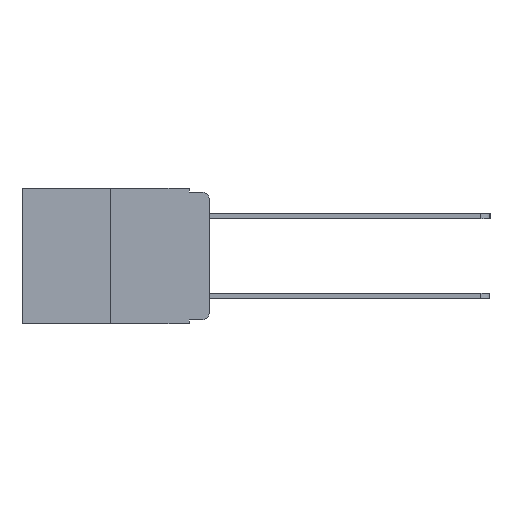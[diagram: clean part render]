
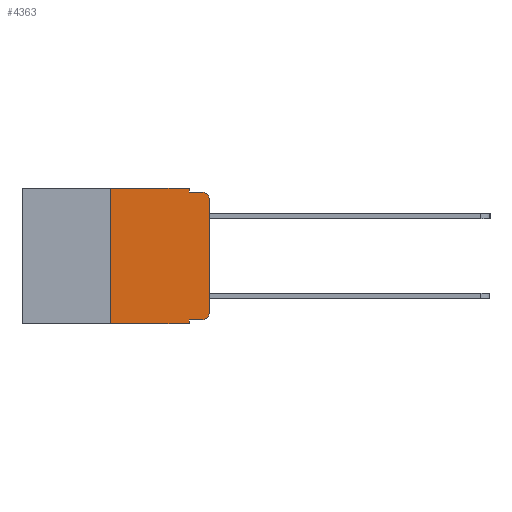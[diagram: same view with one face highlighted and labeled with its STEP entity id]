
A CAD part, left-side view. The second image highlights one B-rep face of the part: STEP entity #4363.
In plain terms, the highlighted planar face has unit normal (-1, 0, 0).
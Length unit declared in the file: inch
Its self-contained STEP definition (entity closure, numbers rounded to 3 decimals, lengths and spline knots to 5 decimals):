
#82 = VECTOR ( 'NONE', #4408, 39.37008 ) ;
#122 = EDGE_CURVE ( 'NONE', #7016, #6286, #2641, .T. ) ;
#457 = ORIENTED_EDGE ( 'NONE', *, *, #4358, .F. ) ;
#758 = ORIENTED_EDGE ( 'NONE', *, *, #6262, .T. ) ;
#801 = EDGE_CURVE ( 'NONE', #7571, #7016, #3825, .T. ) ;
#914 = PLANE ( 'NONE',  #8276 ) ;
#931 = LINE ( 'NONE', #12669, #4138 ) ;
#958 = VECTOR ( 'NONE', #11687, 39.37008 ) ;
#1059 = CARTESIAN_POINT ( 'NONE',  ( 0., 0.02, -0.01 ) ) ;
#1319 = CARTESIAN_POINT ( 'NONE',  ( 0., 0.051, -0.01 ) ) ;
#1342 = CARTESIAN_POINT ( 'NONE',  ( 0., 0.051, 0. ) ) ;
#1504 = EDGE_CURVE ( 'NONE', #7571, #2391, #10440, .T. ) ;
#1581 = CARTESIAN_POINT ( 'NONE',  ( 0., 0.051, -0.333 ) ) ;
#1726 = CARTESIAN_POINT ( 'NONE',  ( 0., 0.02, -0.333 ) ) ;
#2180 = CARTESIAN_POINT ( 'NONE',  ( 0., 0.051, -0.333 ) ) ;
#2243 = EDGE_CURVE ( 'NONE', #11207, #2372, #931, .T. ) ;
#2277 = ORIENTED_EDGE ( 'NONE', *, *, #5172, .T. ) ;
#2372 = VERTEX_POINT ( 'NONE', #4711 ) ;
#2391 = VERTEX_POINT ( 'NONE', #11689 ) ;
#2641 = CIRCLE ( 'NONE', #10747, 0.02 ) ;
#2781 = VECTOR ( 'NONE', #5184, 39.37008 ) ;
#2895 = LINE ( 'NONE', #3265, #82 ) ;
#2938 = ORIENTED_EDGE ( 'NONE', *, *, #2961, .F. ) ;
#2961 = EDGE_CURVE ( 'NONE', #12377, #11466, #12189, .T. ) ;
#3074 = DIRECTION ( 'NONE',  ( 1., 0., 0. ) ) ;
#3123 = DIRECTION ( 'NONE',  ( 0., 0., -1. ) ) ;
#3153 = DIRECTION ( 'NONE',  ( -1., 0., 0. ) ) ;
#3265 = CARTESIAN_POINT ( 'NONE',  ( 0., 0., 0. ) ) ;
#3700 = EDGE_CURVE ( 'NONE', #11466, #9908, #11582, .T. ) ;
#3782 = VECTOR ( 'NONE', #8153, 39.37008 ) ;
#3808 = CARTESIAN_POINT ( 'NONE',  ( 0., 0., -0.313 ) ) ;
#3825 = LINE ( 'NONE', #2180, #958 ) ;
#3977 = AXIS2_PLACEMENT_3D ( 'NONE', #5525, #12126, #6501 ) ;
#4138 = VECTOR ( 'NONE', #12748, 39.37008 ) ;
#4358 = EDGE_CURVE ( 'NONE', #2372, #12377, #11291, .T. ) ;
#4363 = ADVANCED_FACE ( 'NONE', ( #6256 ), #914, .F. ) ;
#4408 = DIRECTION ( 'NONE',  ( 0., 0., 1. ) ) ;
#4439 = EDGE_CURVE ( 'NONE', #6180, #9908, #9840, .T. ) ;
#4711 = CARTESIAN_POINT ( 'NONE',  ( 0., 0.25, 0. ) ) ;
#5172 = EDGE_CURVE ( 'NONE', #6286, #6180, #2895, .T. ) ;
#5175 = ORIENTED_EDGE ( 'NONE', *, *, #4439, .T. ) ;
#5184 = DIRECTION ( 'NONE',  ( 0., 0., -1. ) ) ;
#5523 = ORIENTED_EDGE ( 'NONE', *, *, #3700, .F. ) ;
#5525 = CARTESIAN_POINT ( 'NONE',  ( 0., 0.02, -0.03 ) ) ;
#5952 = CARTESIAN_POINT ( 'NONE',  ( 0., 0.051, 0. ) ) ;
#6126 = ORIENTED_EDGE ( 'NONE', *, *, #2243, .F. ) ;
#6180 = VERTEX_POINT ( 'NONE', #8724 ) ;
#6256 = FACE_OUTER_BOUND ( 'NONE', #7578, .T. ) ;
#6262 = EDGE_CURVE ( 'NONE', #11207, #2391, #12689, .T. ) ;
#6286 = VERTEX_POINT ( 'NONE', #3808 ) ;
#6501 = DIRECTION ( 'NONE',  ( 0., 0., -1. ) ) ;
#7016 = VERTEX_POINT ( 'NONE', #1726 ) ;
#7571 = VERTEX_POINT ( 'NONE', #1581 ) ;
#7578 = EDGE_LOOP ( 'NONE', ( #2277, #5175, #5523, #2938, #457, #6126, #758, #8966, #11445, #9286 ) ) ;
#8153 = DIRECTION ( 'NONE',  ( 0., -1., 0. ) ) ;
#8276 = AXIS2_PLACEMENT_3D ( 'NONE', #10955, #3074, #10071 ) ;
#8724 = CARTESIAN_POINT ( 'NONE',  ( 0., 0., -0.03 ) ) ;
#8803 = CARTESIAN_POINT ( 'NONE',  ( 0., 0.473, -0.343 ) ) ;
#8966 = ORIENTED_EDGE ( 'NONE', *, *, #1504, .F. ) ;
#9110 = VECTOR ( 'NONE', #10825, 39.37008 ) ;
#9286 = ORIENTED_EDGE ( 'NONE', *, *, #122, .T. ) ;
#9521 = CARTESIAN_POINT ( 'NONE',  ( 0., 0.051, 0. ) ) ;
#9561 = DIRECTION ( 'NONE',  ( 0., 0., -1. ) ) ;
#9735 = VECTOR ( 'NONE', #9561, 39.37008 ) ;
#9840 = CIRCLE ( 'NONE', #3977, 0.02 ) ;
#9906 = CARTESIAN_POINT ( 'NONE',  ( 0., 0.051, -0.01 ) ) ;
#9908 = VERTEX_POINT ( 'NONE', #1059 ) ;
#10071 = DIRECTION ( 'NONE',  ( 0., 0., -1. ) ) ;
#10236 = VECTOR ( 'NONE', #10681, 39.37008 ) ;
#10440 = LINE ( 'NONE', #5952, #2781 ) ;
#10590 = CARTESIAN_POINT ( 'NONE',  ( 0., 0.02, -0.313 ) ) ;
#10681 = DIRECTION ( 'NONE',  ( 0., -1., 0. ) ) ;
#10747 = AXIS2_PLACEMENT_3D ( 'NONE', #10590, #3153, #3123 ) ;
#10825 = DIRECTION ( 'NONE',  ( 0., -1., 0. ) ) ;
#10955 = CARTESIAN_POINT ( 'NONE',  ( 0., 0.473, 0. ) ) ;
#11069 = CARTESIAN_POINT ( 'NONE',  ( 0., 0.25, -0.343 ) ) ;
#11207 = VERTEX_POINT ( 'NONE', #11069 ) ;
#11291 = LINE ( 'NONE', #12822, #3782 ) ;
#11445 = ORIENTED_EDGE ( 'NONE', *, *, #801, .T. ) ;
#11466 = VERTEX_POINT ( 'NONE', #1319 ) ;
#11582 = LINE ( 'NONE', #9906, #9110 ) ;
#11687 = DIRECTION ( 'NONE',  ( 0., -1., 0. ) ) ;
#11689 = CARTESIAN_POINT ( 'NONE',  ( 0., 0.051, -0.343 ) ) ;
#12126 = DIRECTION ( 'NONE',  ( -1., 0., 0. ) ) ;
#12189 = LINE ( 'NONE', #9521, #9735 ) ;
#12377 = VERTEX_POINT ( 'NONE', #1342 ) ;
#12669 = CARTESIAN_POINT ( 'NONE',  ( 0., 0.25, 0. ) ) ;
#12689 = LINE ( 'NONE', #8803, #10236 ) ;
#12748 = DIRECTION ( 'NONE',  ( 0., 0., 1. ) ) ;
#12822 = CARTESIAN_POINT ( 'NONE',  ( 0., 0.473, 0. ) ) ;
